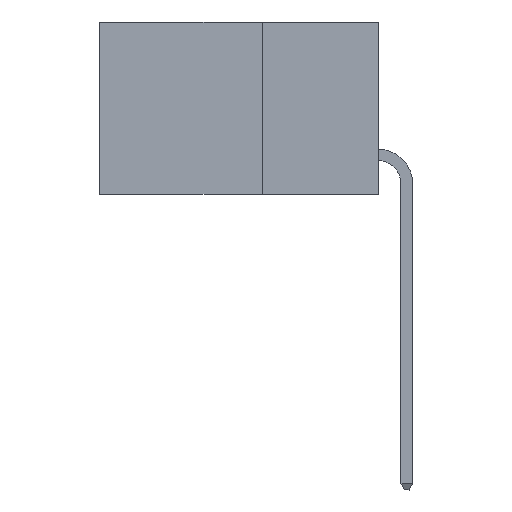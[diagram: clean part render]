
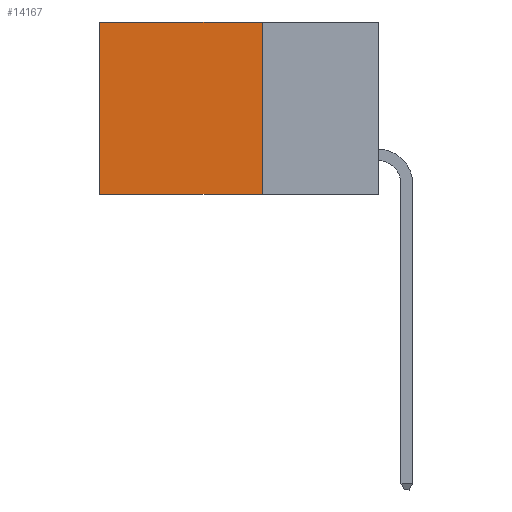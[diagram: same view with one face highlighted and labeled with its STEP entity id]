
A CAD part, left-side view. The second image highlights one B-rep face of the part: STEP entity #14167.
In plain terms, the highlighted planar face has unit normal (-1, 0, 0).
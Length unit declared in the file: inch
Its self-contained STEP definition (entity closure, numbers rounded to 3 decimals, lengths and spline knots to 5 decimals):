
#148 = EDGE_CURVE ( 'NONE', #7538, #18774, #10458, .T. ) ;
#351 = DIRECTION ( 'NONE',  ( 0., 1., 0. ) ) ;
#1113 = ORIENTED_EDGE ( 'NONE', *, *, #12457, .T. ) ;
#1139 = LINE ( 'NONE', #13697, #10810 ) ;
#1311 = CARTESIAN_POINT ( 'NONE',  ( 0.298, 0.25, -0.37 ) ) ;
#1917 = DIRECTION ( 'NONE',  ( 0., 0., -1. ) ) ;
#3297 = LINE ( 'NONE', #15409, #7090 ) ;
#4389 = VECTOR ( 'NONE', #15026, 39.37008 ) ;
#6436 = PLANE ( 'NONE',  #16371 ) ;
#6878 = VERTEX_POINT ( 'NONE', #7148 ) ;
#7064 = CARTESIAN_POINT ( 'NONE',  ( 0.298, 0.25, -0.37 ) ) ;
#7090 = VECTOR ( 'NONE', #351, 39.37008 ) ;
#7148 = CARTESIAN_POINT ( 'NONE',  ( 0.298, 0.25, 0. ) ) ;
#7538 = VERTEX_POINT ( 'NONE', #7064 ) ;
#7549 = DIRECTION ( 'NONE',  ( 0., 0., -1. ) ) ;
#8226 = CARTESIAN_POINT ( 'NONE',  ( 0.298, 0.6, 0. ) ) ;
#8549 = EDGE_LOOP ( 'NONE', ( #1113, #18015, #16969, #17055 ) ) ;
#9496 = DIRECTION ( 'NONE',  ( 0., 0., -1. ) ) ;
#10458 = LINE ( 'NONE', #1311, #4389 ) ;
#10810 = VECTOR ( 'NONE', #7549, 39.37008 ) ;
#11272 = CARTESIAN_POINT ( 'NONE',  ( 0.298, 0.6, -0.37 ) ) ;
#11383 = EDGE_CURVE ( 'NONE', #6878, #11481, #3297, .T. ) ;
#11481 = VERTEX_POINT ( 'NONE', #8226 ) ;
#12457 = EDGE_CURVE ( 'NONE', #11481, #18774, #14078, .T. ) ;
#12512 = DIRECTION ( 'NONE',  ( 1., 0., 0. ) ) ;
#13697 = CARTESIAN_POINT ( 'NONE',  ( 0.298, 0.25, 0. ) ) ;
#14075 = CARTESIAN_POINT ( 'NONE',  ( 0.298, 0.6, 0. ) ) ;
#14078 = LINE ( 'NONE', #14075, #16982 ) ;
#14091 = CARTESIAN_POINT ( 'NONE',  ( 0.298, 0.25, 0. ) ) ;
#14167 = ADVANCED_FACE ( 'NONE', ( #18557 ), #6436, .F. ) ;
#15026 = DIRECTION ( 'NONE',  ( 0., 1., 0. ) ) ;
#15409 = CARTESIAN_POINT ( 'NONE',  ( 0.298, 0.25, 0. ) ) ;
#16371 = AXIS2_PLACEMENT_3D ( 'NONE', #14091, #12512, #9496 ) ;
#16969 = ORIENTED_EDGE ( 'NONE', *, *, #17595, .F. ) ;
#16982 = VECTOR ( 'NONE', #1917, 39.37008 ) ;
#17055 = ORIENTED_EDGE ( 'NONE', *, *, #11383, .T. ) ;
#17595 = EDGE_CURVE ( 'NONE', #6878, #7538, #1139, .T. ) ;
#18015 = ORIENTED_EDGE ( 'NONE', *, *, #148, .F. ) ;
#18557 = FACE_OUTER_BOUND ( 'NONE', #8549, .T. ) ;
#18774 = VERTEX_POINT ( 'NONE', #11272 ) ;
